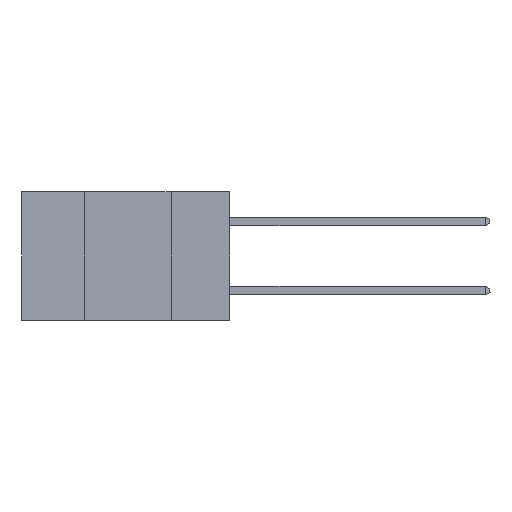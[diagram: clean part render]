
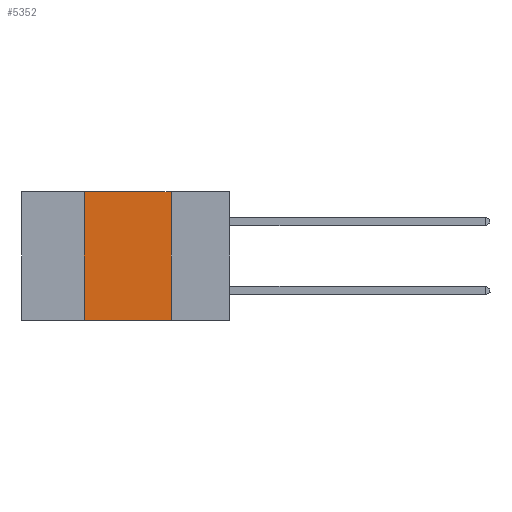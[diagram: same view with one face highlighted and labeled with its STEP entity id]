
A CAD part, left-side view. The second image highlights one B-rep face of the part: STEP entity #5352.
In plain terms, the highlighted planar face has unit normal (-1, 0, 0).
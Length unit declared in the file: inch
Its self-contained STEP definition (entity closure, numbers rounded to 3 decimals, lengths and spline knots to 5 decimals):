
#325 = DIRECTION ( 'NONE',  ( 0., -1., 0. ) ) ;
#1298 = LINE ( 'NONE', #8203, #24607 ) ;
#1300 = EDGE_CURVE ( 'NONE', #18620, #8724, #18090, .T. ) ;
#2135 = VERTEX_POINT ( 'NONE', #12607 ) ;
#3755 = CARTESIAN_POINT ( 'NONE',  ( 0., 0.6, 0. ) ) ;
#4617 = DIRECTION ( 'NONE',  ( 1., 0., 0. ) ) ;
#5352 = ADVANCED_FACE ( 'NONE', ( #16027 ), #17924, .F. ) ;
#5543 = CARTESIAN_POINT ( 'NONE',  ( 0., 0.17, 0. ) ) ;
#5926 = EDGE_LOOP ( 'NONE', ( #9162, #8501, #9089, #27024 ) ) ;
#8203 = CARTESIAN_POINT ( 'NONE',  ( 0., 0.42, 0. ) ) ;
#8501 = ORIENTED_EDGE ( 'NONE', *, *, #1300, .F. ) ;
#8517 = LINE ( 'NONE', #5543, #10652 ) ;
#8724 = VERTEX_POINT ( 'NONE', #10791 ) ;
#9089 = ORIENTED_EDGE ( 'NONE', *, *, #29110, .F. ) ;
#9162 = ORIENTED_EDGE ( 'NONE', *, *, #26961, .F. ) ;
#9794 = DIRECTION ( 'NONE',  ( 0., 0., -1. ) ) ;
#9887 = AXIS2_PLACEMENT_3D ( 'NONE', #13382, #4617, #13565 ) ;
#10366 = VECTOR ( 'NONE', #21620, 39.37008 ) ;
#10652 = VECTOR ( 'NONE', #9794, 39.37008 ) ;
#10791 = CARTESIAN_POINT ( 'NONE',  ( 0., 0.17, 0. ) ) ;
#12488 = CARTESIAN_POINT ( 'NONE',  ( 0., 0.17, -0.37 ) ) ;
#12607 = CARTESIAN_POINT ( 'NONE',  ( 0., 0.42, -0.37 ) ) ;
#12722 = DIRECTION ( 'NONE',  ( 0., 0., 1. ) ) ;
#13264 = CARTESIAN_POINT ( 'NONE',  ( 0., 0.42, 0. ) ) ;
#13382 = CARTESIAN_POINT ( 'NONE',  ( 0., 0.6, 0. ) ) ;
#13565 = DIRECTION ( 'NONE',  ( 0., 0., -1. ) ) ;
#16027 = FACE_OUTER_BOUND ( 'NONE', #5926, .T. ) ;
#17883 = LINE ( 'NONE', #22825, #22828 ) ;
#17924 = PLANE ( 'NONE',  #9887 ) ;
#18090 = LINE ( 'NONE', #3755, #10366 ) ;
#18620 = VERTEX_POINT ( 'NONE', #13264 ) ;
#19704 = VERTEX_POINT ( 'NONE', #12488 ) ;
#21620 = DIRECTION ( 'NONE',  ( 0., -1., 0. ) ) ;
#22825 = CARTESIAN_POINT ( 'NONE',  ( 0., 0.6, -0.37 ) ) ;
#22828 = VECTOR ( 'NONE', #325, 39.37008 ) ;
#23078 = EDGE_CURVE ( 'NONE', #2135, #19704, #17883, .T. ) ;
#24607 = VECTOR ( 'NONE', #12722, 39.37008 ) ;
#26961 = EDGE_CURVE ( 'NONE', #8724, #19704, #8517, .T. ) ;
#27024 = ORIENTED_EDGE ( 'NONE', *, *, #23078, .T. ) ;
#29110 = EDGE_CURVE ( 'NONE', #2135, #18620, #1298, .T. ) ;
